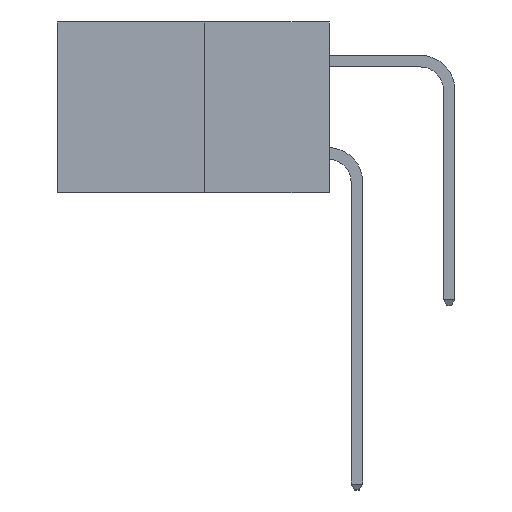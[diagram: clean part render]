
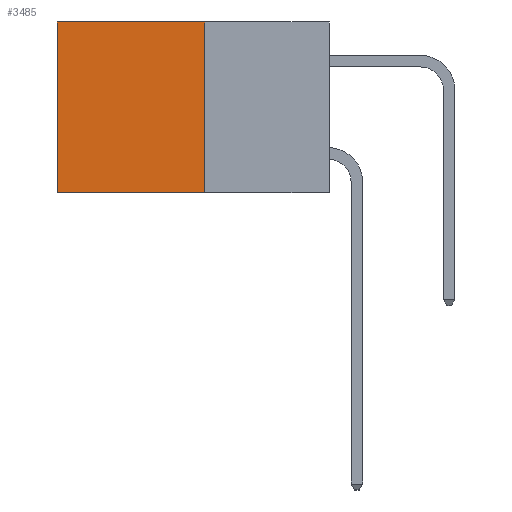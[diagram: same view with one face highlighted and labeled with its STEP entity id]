
A CAD part, left-side view. The second image highlights one B-rep face of the part: STEP entity #3485.
In plain terms, the highlighted planar face has unit normal (-1, 0, 0).
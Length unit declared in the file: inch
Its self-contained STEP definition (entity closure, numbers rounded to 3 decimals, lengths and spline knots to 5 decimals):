
#389 = LINE ( 'NONE', #748, #8364 ) ;
#720 = FACE_OUTER_BOUND ( 'NONE', #3227, .T. ) ;
#748 = CARTESIAN_POINT ( 'NONE',  ( 0.277, 0.59, -0.37 ) ) ;
#783 = DIRECTION ( 'NONE',  ( 0., 0., -1. ) ) ;
#814 = AXIS2_PLACEMENT_3D ( 'NONE', #8922, #5770, #8447 ) ;
#938 = ORIENTED_EDGE ( 'NONE', *, *, #4734, .T. ) ;
#1395 = CARTESIAN_POINT ( 'NONE',  ( 0.277, 0.27, -0.37 ) ) ;
#1789 = EDGE_CURVE ( 'NONE', #9457, #2394, #8012, .T. ) ;
#2394 = VERTEX_POINT ( 'NONE', #5509 ) ;
#2887 = DIRECTION ( 'NONE',  ( 0., 1., 0. ) ) ;
#3012 = CARTESIAN_POINT ( 'NONE',  ( 0.277, 0.27, 0. ) ) ;
#3139 = ORIENTED_EDGE ( 'NONE', *, *, #4038, .F. ) ;
#3227 = EDGE_LOOP ( 'NONE', ( #5539, #6377, #3139, #938 ) ) ;
#3485 = ADVANCED_FACE ( 'NONE', ( #720 ), #7697, .F. ) ;
#3744 = VECTOR ( 'NONE', #6667, 39.37008 ) ;
#4038 = EDGE_CURVE ( 'NONE', #5961, #9457, #5689, .T. ) ;
#4451 = VERTEX_POINT ( 'NONE', #6727 ) ;
#4734 = EDGE_CURVE ( 'NONE', #5961, #4451, #5019, .T. ) ;
#5019 = LINE ( 'NONE', #3012, #8776 ) ;
#5037 = EDGE_CURVE ( 'NONE', #4451, #2394, #389, .T. ) ;
#5509 = CARTESIAN_POINT ( 'NONE',  ( 0.277, 0.59, -0.37 ) ) ;
#5539 = ORIENTED_EDGE ( 'NONE', *, *, #5037, .T. ) ;
#5689 = LINE ( 'NONE', #6747, #3744 ) ;
#5770 = DIRECTION ( 'NONE',  ( 1., 0., 0. ) ) ;
#5961 = VERTEX_POINT ( 'NONE', #8180 ) ;
#6377 = ORIENTED_EDGE ( 'NONE', *, *, #1789, .F. ) ;
#6667 = DIRECTION ( 'NONE',  ( 0., 0., -1. ) ) ;
#6727 = CARTESIAN_POINT ( 'NONE',  ( 0.277, 0.59, 0. ) ) ;
#6747 = CARTESIAN_POINT ( 'NONE',  ( 0.277, 0.27, -0.37 ) ) ;
#7372 = CARTESIAN_POINT ( 'NONE',  ( 0.277, 0.27, -0.37 ) ) ;
#7697 = PLANE ( 'NONE',  #814 ) ;
#8012 = LINE ( 'NONE', #1395, #8241 ) ;
#8180 = CARTESIAN_POINT ( 'NONE',  ( 0.277, 0.27, 0. ) ) ;
#8241 = VECTOR ( 'NONE', #8819, 39.37008 ) ;
#8364 = VECTOR ( 'NONE', #783, 39.37008 ) ;
#8447 = DIRECTION ( 'NONE',  ( 0., 0., -1. ) ) ;
#8776 = VECTOR ( 'NONE', #2887, 39.37008 ) ;
#8819 = DIRECTION ( 'NONE',  ( 0., 1., 0. ) ) ;
#8922 = CARTESIAN_POINT ( 'NONE',  ( 0.277, 0.27, -0.37 ) ) ;
#9457 = VERTEX_POINT ( 'NONE', #7372 ) ;
